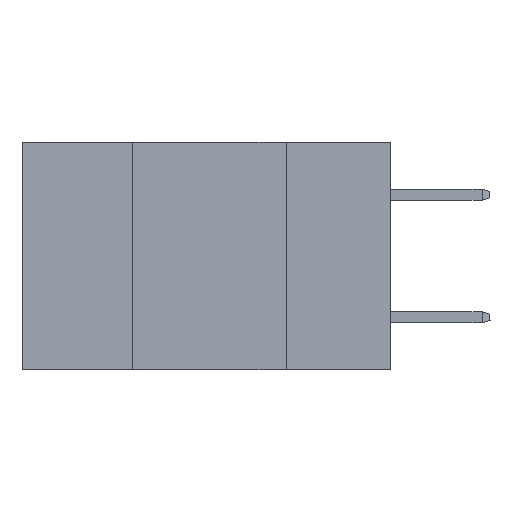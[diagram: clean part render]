
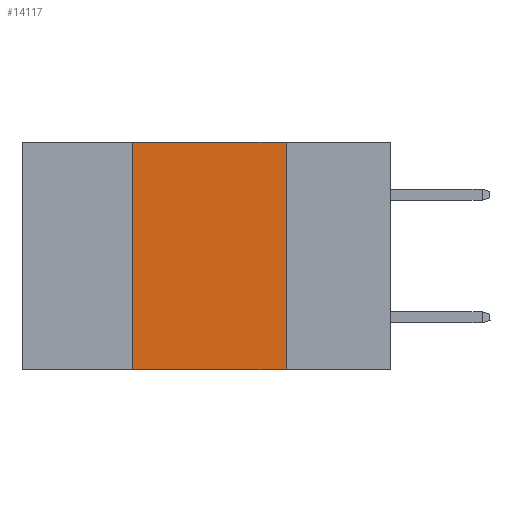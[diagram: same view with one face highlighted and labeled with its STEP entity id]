
A CAD part, left-side view. The second image highlights one B-rep face of the part: STEP entity #14117.
In plain terms, the highlighted planar face has unit normal (-1, 0, 0).
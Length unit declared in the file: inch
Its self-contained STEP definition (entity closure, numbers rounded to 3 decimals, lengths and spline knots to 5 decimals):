
#103 = EDGE_CURVE ( 'NONE', #2981, #24682, #25997, .T. ) ;
#666 = VERTEX_POINT ( 'NONE', #4962 ) ;
#1177 = DIRECTION ( 'NONE',  ( 0., -1., 0. ) ) ;
#1480 = LINE ( 'NONE', #10223, #1844 ) ;
#1844 = VECTOR ( 'NONE', #1177, 39.37008 ) ;
#2263 = CARTESIAN_POINT ( 'NONE',  ( 0., 0.42, 0. ) ) ;
#2981 = VERTEX_POINT ( 'NONE', #27285 ) ;
#4962 = CARTESIAN_POINT ( 'NONE',  ( 0., 0.42, 0. ) ) ;
#7924 = VERTEX_POINT ( 'NONE', #30372 ) ;
#8291 = LINE ( 'NONE', #2263, #16765 ) ;
#10223 = CARTESIAN_POINT ( 'NONE',  ( 0., 0.6, 0. ) ) ;
#10641 = EDGE_CURVE ( 'NONE', #666, #7924, #1480, .T. ) ;
#12100 = CARTESIAN_POINT ( 'NONE',  ( 0., 0.6, 0. ) ) ;
#12199 = DIRECTION ( 'NONE',  ( 0., 0., -1. ) ) ;
#12270 = EDGE_CURVE ( 'NONE', #2981, #666, #8291, .T. ) ;
#12768 = DIRECTION ( 'NONE',  ( 0., 0., 1. ) ) ;
#14117 = ADVANCED_FACE ( 'NONE', ( #14205 ), #29119, .F. ) ;
#14205 = FACE_OUTER_BOUND ( 'NONE', #15187, .T. ) ;
#14384 = LINE ( 'NONE', #31496, #27446 ) ;
#14563 = DIRECTION ( 'NONE',  ( 1., 0., 0. ) ) ;
#15187 = EDGE_LOOP ( 'NONE', ( #23908, #21679, #24010, #31234 ) ) ;
#16765 = VECTOR ( 'NONE', #12768, 39.37008 ) ;
#18312 = VECTOR ( 'NONE', #28711, 39.37008 ) ;
#18785 = DIRECTION ( 'NONE',  ( 0., 0., -1. ) ) ;
#20433 = EDGE_CURVE ( 'NONE', #7924, #24682, #14384, .T. ) ;
#20979 = AXIS2_PLACEMENT_3D ( 'NONE', #12100, #14563, #12199 ) ;
#21679 = ORIENTED_EDGE ( 'NONE', *, *, #10641, .F. ) ;
#23908 = ORIENTED_EDGE ( 'NONE', *, *, #20433, .F. ) ;
#24010 = ORIENTED_EDGE ( 'NONE', *, *, #12270, .F. ) ;
#24682 = VERTEX_POINT ( 'NONE', #24808 ) ;
#24808 = CARTESIAN_POINT ( 'NONE',  ( 0., 0.17, -0.37 ) ) ;
#25997 = LINE ( 'NONE', #28938, #18312 ) ;
#27285 = CARTESIAN_POINT ( 'NONE',  ( 0., 0.42, -0.37 ) ) ;
#27446 = VECTOR ( 'NONE', #18785, 39.37008 ) ;
#28711 = DIRECTION ( 'NONE',  ( 0., -1., 0. ) ) ;
#28938 = CARTESIAN_POINT ( 'NONE',  ( 0., 0.6, -0.37 ) ) ;
#29119 = PLANE ( 'NONE',  #20979 ) ;
#30372 = CARTESIAN_POINT ( 'NONE',  ( 0., 0.17, 0. ) ) ;
#31234 = ORIENTED_EDGE ( 'NONE', *, *, #103, .T. ) ;
#31496 = CARTESIAN_POINT ( 'NONE',  ( 0., 0.17, 0. ) ) ;
